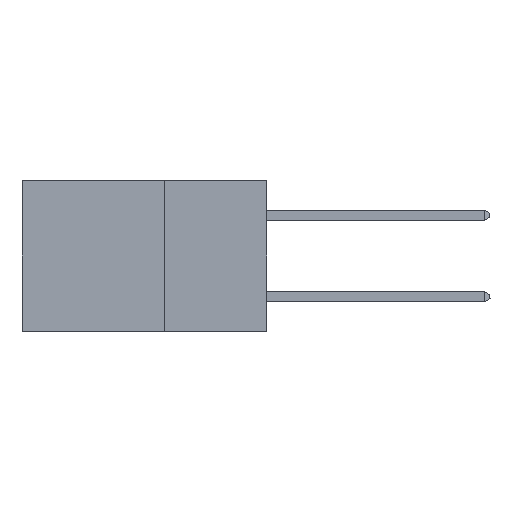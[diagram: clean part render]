
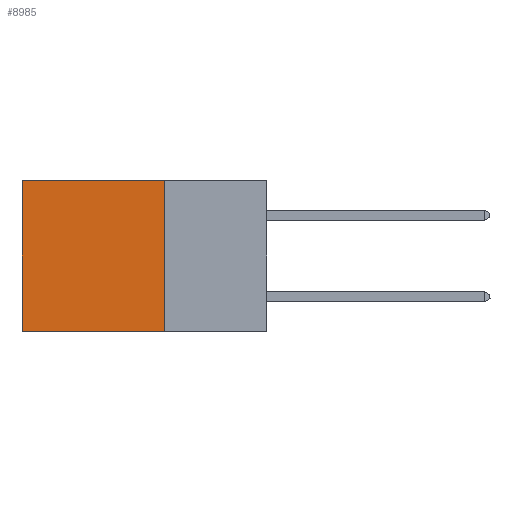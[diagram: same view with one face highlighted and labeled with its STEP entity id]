
A CAD part, left-side view. The second image highlights one B-rep face of the part: STEP entity #8985.
In plain terms, the highlighted planar face has unit normal (-1, 0, 0).
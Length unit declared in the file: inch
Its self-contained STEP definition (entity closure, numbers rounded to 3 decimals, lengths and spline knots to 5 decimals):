
#1409 = EDGE_CURVE ( 'NONE', #29690, #19999, #30491, .T. ) ;
#1706 = ORIENTED_EDGE ( 'NONE', *, *, #14573, .F. ) ;
#2961 = VECTOR ( 'NONE', #3667, 39.37008 ) ;
#3667 = DIRECTION ( 'NONE',  ( 0., 1., 0. ) ) ;
#4832 = VERTEX_POINT ( 'NONE', #13612 ) ;
#8251 = EDGE_CURVE ( 'NONE', #4832, #29690, #22432, .T. ) ;
#8985 = ADVANCED_FACE ( 'NONE', ( #28292 ), #17993, .F. ) ;
#9233 = CARTESIAN_POINT ( 'NONE',  ( 0.2875, 0.6, 0. ) ) ;
#10031 = VERTEX_POINT ( 'NONE', #19275 ) ;
#12308 = ORIENTED_EDGE ( 'NONE', *, *, #22436, .F. ) ;
#13612 = CARTESIAN_POINT ( 'NONE',  ( 0.2875, 0.25, 0. ) ) ;
#13775 = DIRECTION ( 'NONE',  ( 0., 0., -1. ) ) ;
#14573 = EDGE_CURVE ( 'NONE', #4832, #10031, #32988, .T. ) ;
#14907 = DIRECTION ( 'NONE',  ( 0., 1., 0. ) ) ;
#17993 = PLANE ( 'NONE',  #20083 ) ;
#18125 = CARTESIAN_POINT ( 'NONE',  ( 0.2875, 0.25, 0. ) ) ;
#19275 = CARTESIAN_POINT ( 'NONE',  ( 0.2875, 0.25, -0.37 ) ) ;
#19999 = VERTEX_POINT ( 'NONE', #36638 ) ;
#20083 = AXIS2_PLACEMENT_3D ( 'NONE', #18125, #39990, #30905 ) ;
#21170 = VECTOR ( 'NONE', #13775, 39.37008 ) ;
#22432 = LINE ( 'NONE', #39749, #24914 ) ;
#22436 = EDGE_CURVE ( 'NONE', #10031, #19999, #33903, .T. ) ;
#22865 = CARTESIAN_POINT ( 'NONE',  ( 0.2875, 0.25, -0.37 ) ) ;
#23604 = ORIENTED_EDGE ( 'NONE', *, *, #8251, .T. ) ;
#24914 = VECTOR ( 'NONE', #14907, 39.37008 ) ;
#25330 = DIRECTION ( 'NONE',  ( 0., 0., -1. ) ) ;
#27244 = EDGE_LOOP ( 'NONE', ( #32993, #12308, #1706, #23604 ) ) ;
#28292 = FACE_OUTER_BOUND ( 'NONE', #27244, .T. ) ;
#29690 = VERTEX_POINT ( 'NONE', #38802 ) ;
#30491 = LINE ( 'NONE', #9233, #34422 ) ;
#30905 = DIRECTION ( 'NONE',  ( 0., 0., -1. ) ) ;
#32988 = LINE ( 'NONE', #35609, #21170 ) ;
#32993 = ORIENTED_EDGE ( 'NONE', *, *, #1409, .T. ) ;
#33903 = LINE ( 'NONE', #22865, #2961 ) ;
#34422 = VECTOR ( 'NONE', #25330, 39.37008 ) ;
#35609 = CARTESIAN_POINT ( 'NONE',  ( 0.2875, 0.25, 0. ) ) ;
#36638 = CARTESIAN_POINT ( 'NONE',  ( 0.2875, 0.6, -0.37 ) ) ;
#38802 = CARTESIAN_POINT ( 'NONE',  ( 0.2875, 0.6, 0. ) ) ;
#39749 = CARTESIAN_POINT ( 'NONE',  ( 0.2875, 0.25, 0. ) ) ;
#39990 = DIRECTION ( 'NONE',  ( 1., 0., 0. ) ) ;
